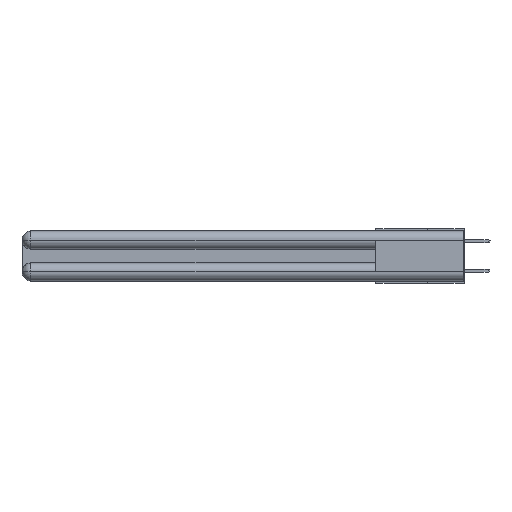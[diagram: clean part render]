
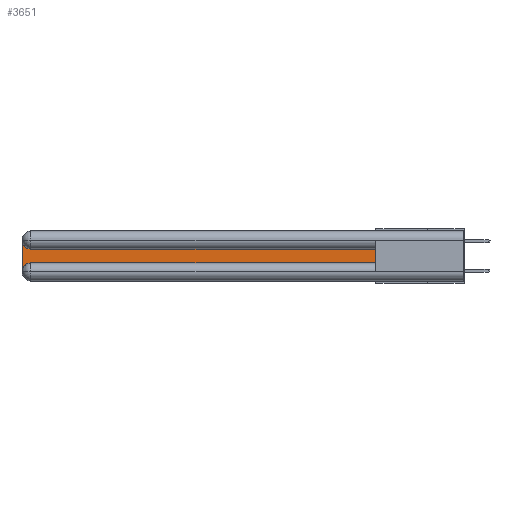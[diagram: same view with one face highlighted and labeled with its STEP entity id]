
A CAD part, left-side view. The second image highlights one B-rep face of the part: STEP entity #3651.
In plain terms, the highlighted planar face has unit normal (-1, 0, 0).
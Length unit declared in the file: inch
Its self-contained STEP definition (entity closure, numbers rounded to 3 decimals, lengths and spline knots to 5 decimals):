
#526 = EDGE_CURVE ( 'NONE', #18075, #11475, #8467, .T. ) ;
#625 = CIRCLE ( 'NONE', #27355, 0.06 ) ;
#761 = EDGE_CURVE ( 'NONE', #14164, #16107, #7328, .T. ) ;
#2818 = CARTESIAN_POINT ( 'NONE',  ( 0.075, 3., -0.0625 ) ) ;
#3084 = CARTESIAN_POINT ( 'NONE',  ( 0.075, 0.6, -0.1225 ) ) ;
#3384 = EDGE_CURVE ( 'NONE', #11475, #14164, #625, .T. ) ;
#3651 = ADVANCED_FACE ( 'NONE', ( #15501 ), #21683, .F. ) ;
#4053 = LINE ( 'NONE', #16620, #27039 ) ;
#4829 = ORIENTED_EDGE ( 'NONE', *, *, #7780, .T. ) ;
#5161 = ORIENTED_EDGE ( 'NONE', *, *, #3384, .T. ) ;
#5364 = CARTESIAN_POINT ( 'NONE',  ( 0.075, 0.6, -0.2175 ) ) ;
#5406 = DIRECTION ( 'NONE',  ( 0., 0., -1. ) ) ;
#5780 = CARTESIAN_POINT ( 'NONE',  ( 0.075, 2.94, -0.1225 ) ) ;
#6515 = LINE ( 'NONE', #5364, #26690 ) ;
#7328 = LINE ( 'NONE', #17307, #26817 ) ;
#7780 = EDGE_CURVE ( 'NONE', #16107, #19191, #6515, .T. ) ;
#7934 = DIRECTION ( 'NONE',  ( 0., 0., -1. ) ) ;
#8058 = DIRECTION ( 'NONE',  ( 1., 0., 0. ) ) ;
#8467 = LINE ( 'NONE', #14083, #16796 ) ;
#8564 = ORIENTED_EDGE ( 'NONE', *, *, #526, .T. ) ;
#8666 = EDGE_CURVE ( 'NONE', #19191, #24443, #4053, .T. ) ;
#9831 = DIRECTION ( 'NONE',  ( 0., 0., 1. ) ) ;
#10171 = CARTESIAN_POINT ( 'NONE',  ( 0.075, 2.94, -0.2775 ) ) ;
#11475 = VERTEX_POINT ( 'NONE', #18833 ) ;
#12520 = DIRECTION ( 'NONE',  ( 1., 0., 0. ) ) ;
#14083 = CARTESIAN_POINT ( 'NONE',  ( 0.075, 3., -0.2175 ) ) ;
#14164 = VERTEX_POINT ( 'NONE', #16741 ) ;
#15291 = ORIENTED_EDGE ( 'NONE', *, *, #8666, .T. ) ;
#15501 = FACE_OUTER_BOUND ( 'NONE', #24413, .T. ) ;
#15514 = AXIS2_PLACEMENT_3D ( 'NONE', #19050, #8058, #28157 ) ;
#16018 = EDGE_CURVE ( 'NONE', #24443, #18075, #22697, .T. ) ;
#16107 = VERTEX_POINT ( 'NONE', #28452 ) ;
#16620 = CARTESIAN_POINT ( 'NONE',  ( 0.075, 0.6, -0.1225 ) ) ;
#16741 = CARTESIAN_POINT ( 'NONE',  ( 0.075, 2.94, -0.2175 ) ) ;
#16796 = VECTOR ( 'NONE', #27632, 39.37008 ) ;
#17307 = CARTESIAN_POINT ( 'NONE',  ( 0.075, 0.6, -0.2175 ) ) ;
#18075 = VERTEX_POINT ( 'NONE', #2818 ) ;
#18833 = CARTESIAN_POINT ( 'NONE',  ( 0.075, 3., -0.2775 ) ) ;
#19050 = CARTESIAN_POINT ( 'NONE',  ( 0.075, 2.94, -0.0625 ) ) ;
#19191 = VERTEX_POINT ( 'NONE', #3084 ) ;
#21305 = CARTESIAN_POINT ( 'NONE',  ( 0.075, 3., -0.1225 ) ) ;
#21566 = AXIS2_PLACEMENT_3D ( 'NONE', #21305, #12520, #7934 ) ;
#21683 = PLANE ( 'NONE',  #21566 ) ;
#21877 = ORIENTED_EDGE ( 'NONE', *, *, #16018, .T. ) ;
#22697 = CIRCLE ( 'NONE', #15514, 0.06 ) ;
#22989 = ORIENTED_EDGE ( 'NONE', *, *, #761, .T. ) ;
#24413 = EDGE_LOOP ( 'NONE', ( #15291, #21877, #8564, #5161, #22989, #4829 ) ) ;
#24443 = VERTEX_POINT ( 'NONE', #5780 ) ;
#26690 = VECTOR ( 'NONE', #9831, 39.37008 ) ;
#26817 = VECTOR ( 'NONE', #28663, 39.37008 ) ;
#27039 = VECTOR ( 'NONE', #27670, 39.37008 ) ;
#27355 = AXIS2_PLACEMENT_3D ( 'NONE', #10171, #27987, #5406 ) ;
#27632 = DIRECTION ( 'NONE',  ( 0., 0., -1. ) ) ;
#27670 = DIRECTION ( 'NONE',  ( 0., 1., 0. ) ) ;
#27987 = DIRECTION ( 'NONE',  ( 1., 0., 0. ) ) ;
#28157 = DIRECTION ( 'NONE',  ( 0., 0., -1. ) ) ;
#28452 = CARTESIAN_POINT ( 'NONE',  ( 0.075, 0.6, -0.2175 ) ) ;
#28663 = DIRECTION ( 'NONE',  ( 0., -1., 0. ) ) ;
